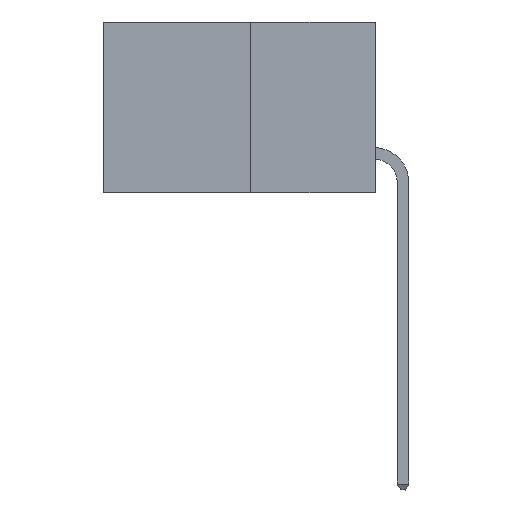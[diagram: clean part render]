
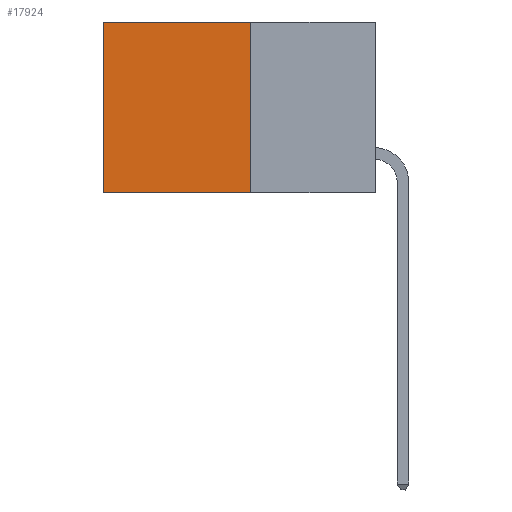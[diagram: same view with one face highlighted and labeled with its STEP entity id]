
A CAD part, left-side view. The second image highlights one B-rep face of the part: STEP entity #17924.
In plain terms, the highlighted planar face has unit normal (-1, 0, 0).
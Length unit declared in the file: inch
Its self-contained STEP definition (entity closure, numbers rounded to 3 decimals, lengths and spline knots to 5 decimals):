
#87 = ORIENTED_EDGE ( 'NONE', *, *, #15563, .T. ) ;
#102 = ORIENTED_EDGE ( 'NONE', *, *, #2014, .F. ) ;
#670 = CARTESIAN_POINT ( 'NONE',  ( 0.277, 0.27, -0.37 ) ) ;
#1808 = CARTESIAN_POINT ( 'NONE',  ( 0.277, 0.27, 0. ) ) ;
#2014 = EDGE_CURVE ( 'NONE', #4099, #7519, #20137, .T. ) ;
#2086 = CARTESIAN_POINT ( 'NONE',  ( 0.277, 0.27, -0.37 ) ) ;
#2124 = CARTESIAN_POINT ( 'NONE',  ( 0.277, 0.27, -0.37 ) ) ;
#2566 = DIRECTION ( 'NONE',  ( 0., 0., -1. ) ) ;
#3010 = ORIENTED_EDGE ( 'NONE', *, *, #19123, .F. ) ;
#3657 = LINE ( 'NONE', #2124, #12551 ) ;
#3777 = PLANE ( 'NONE',  #13435 ) ;
#4099 = VERTEX_POINT ( 'NONE', #6194 ) ;
#5355 = VERTEX_POINT ( 'NONE', #17356 ) ;
#6194 = CARTESIAN_POINT ( 'NONE',  ( 0.277, 0.27, -0.37 ) ) ;
#7519 = VERTEX_POINT ( 'NONE', #16278 ) ;
#9050 = DIRECTION ( 'NONE',  ( 0., 1., 0. ) ) ;
#9787 = EDGE_CURVE ( 'NONE', #17857, #7519, #14658, .T. ) ;
#10251 = VECTOR ( 'NONE', #2566, 39.37008 ) ;
#10313 = CARTESIAN_POINT ( 'NONE',  ( 0.277, 0.59, 0. ) ) ;
#10517 = DIRECTION ( 'NONE',  ( 0., 0., -1. ) ) ;
#11042 = ORIENTED_EDGE ( 'NONE', *, *, #9787, .T. ) ;
#11453 = EDGE_LOOP ( 'NONE', ( #11042, #102, #3010, #87 ) ) ;
#12551 = VECTOR ( 'NONE', #13820, 39.37008 ) ;
#13142 = LINE ( 'NONE', #1808, #16997 ) ;
#13435 = AXIS2_PLACEMENT_3D ( 'NONE', #2086, #20389, #10517 ) ;
#13820 = DIRECTION ( 'NONE',  ( 0., 0., -1. ) ) ;
#14658 = LINE ( 'NONE', #19148, #10251 ) ;
#15461 = FACE_OUTER_BOUND ( 'NONE', #11453, .T. ) ;
#15563 = EDGE_CURVE ( 'NONE', #5355, #17857, #13142, .T. ) ;
#15756 = VECTOR ( 'NONE', #9050, 39.37008 ) ;
#16278 = CARTESIAN_POINT ( 'NONE',  ( 0.277, 0.59, -0.37 ) ) ;
#16997 = VECTOR ( 'NONE', #18472, 39.37008 ) ;
#17356 = CARTESIAN_POINT ( 'NONE',  ( 0.277, 0.27, 0. ) ) ;
#17857 = VERTEX_POINT ( 'NONE', #10313 ) ;
#17924 = ADVANCED_FACE ( 'NONE', ( #15461 ), #3777, .F. ) ;
#18472 = DIRECTION ( 'NONE',  ( 0., 1., 0. ) ) ;
#19123 = EDGE_CURVE ( 'NONE', #5355, #4099, #3657, .T. ) ;
#19148 = CARTESIAN_POINT ( 'NONE',  ( 0.277, 0.59, -0.37 ) ) ;
#20137 = LINE ( 'NONE', #670, #15756 ) ;
#20389 = DIRECTION ( 'NONE',  ( 1., 0., 0. ) ) ;
